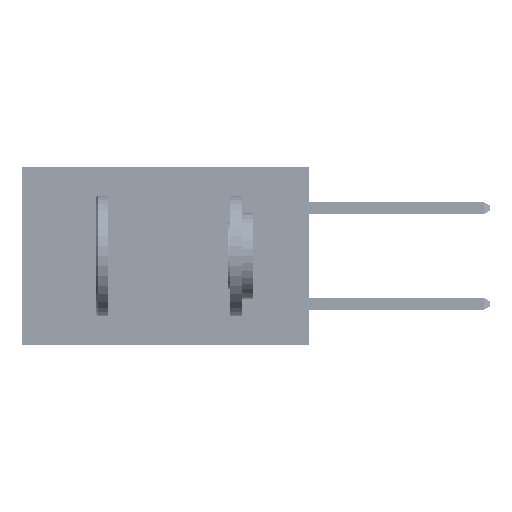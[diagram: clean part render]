
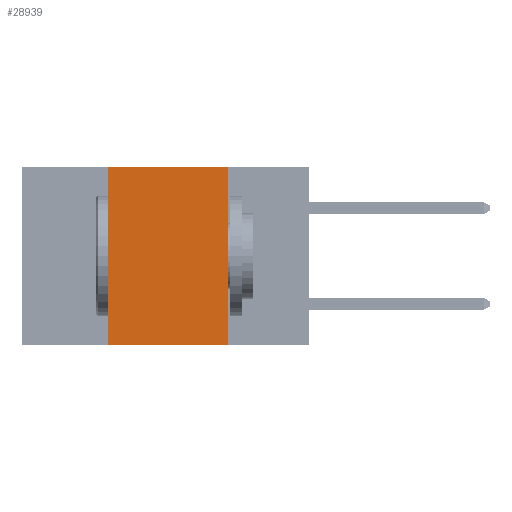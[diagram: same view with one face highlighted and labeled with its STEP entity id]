
A CAD part, left-side view. The second image highlights one B-rep face of the part: STEP entity #28939.
In plain terms, the highlighted planar face has unit normal (-1, 0, 0).
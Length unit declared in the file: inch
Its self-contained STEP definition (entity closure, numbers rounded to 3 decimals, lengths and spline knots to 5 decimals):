
#405 = VECTOR ( 'NONE', #922, 39.37008 ) ;
#922 = DIRECTION ( 'NONE',  ( 0., 0., 1. ) ) ;
#2161 = EDGE_LOOP ( 'NONE', ( #22562, #3399, #42289, #28009 ) ) ;
#2400 = DIRECTION ( 'NONE',  ( 0., -1., 0. ) ) ;
#3399 = ORIENTED_EDGE ( 'NONE', *, *, #45378, .F. ) ;
#3670 = VECTOR ( 'NONE', #2400, 39.37008 ) ;
#4872 = VECTOR ( 'NONE', #13951, 39.37008 ) ;
#6285 = CARTESIAN_POINT ( 'NONE',  ( 0., 0.6, 0. ) ) ;
#7671 = LINE ( 'NONE', #22929, #45826 ) ;
#9110 = AXIS2_PLACEMENT_3D ( 'NONE', #14588, #41474, #18618 ) ;
#10226 = CARTESIAN_POINT ( 'NONE',  ( 0., 0.42, -0.37 ) ) ;
#12044 = CARTESIAN_POINT ( 'NONE',  ( 0., 0.17, -0.37 ) ) ;
#13951 = DIRECTION ( 'NONE',  ( 0., -1., 0. ) ) ;
#14588 = CARTESIAN_POINT ( 'NONE',  ( 0., 0.6, 0. ) ) ;
#14754 = PLANE ( 'NONE',  #9110 ) ;
#15049 = LINE ( 'NONE', #17637, #3670 ) ;
#15059 = LINE ( 'NONE', #6285, #4872 ) ;
#17637 = CARTESIAN_POINT ( 'NONE',  ( 0., 0.6, -0.37 ) ) ;
#18618 = DIRECTION ( 'NONE',  ( 0., 0., -1. ) ) ;
#19259 = DIRECTION ( 'NONE',  ( 0., 0., -1. ) ) ;
#20032 = CARTESIAN_POINT ( 'NONE',  ( 0., 0.42, 0. ) ) ;
#22004 = LINE ( 'NONE', #20032, #405 ) ;
#22562 = ORIENTED_EDGE ( 'NONE', *, *, #41859, .F. ) ;
#22929 = CARTESIAN_POINT ( 'NONE',  ( 0., 0.17, 0. ) ) ;
#23958 = EDGE_CURVE ( 'NONE', #41584, #40954, #22004, .T. ) ;
#27490 = EDGE_CURVE ( 'NONE', #41584, #46346, #15049, .T. ) ;
#28009 = ORIENTED_EDGE ( 'NONE', *, *, #27490, .T. ) ;
#28939 = ADVANCED_FACE ( 'NONE', ( #45161 ), #14754, .F. ) ;
#31730 = CARTESIAN_POINT ( 'NONE',  ( 0., 0.17, 0. ) ) ;
#37484 = CARTESIAN_POINT ( 'NONE',  ( 0., 0.42, 0. ) ) ;
#40954 = VERTEX_POINT ( 'NONE', #37484 ) ;
#41474 = DIRECTION ( 'NONE',  ( 1., 0., 0. ) ) ;
#41584 = VERTEX_POINT ( 'NONE', #10226 ) ;
#41859 = EDGE_CURVE ( 'NONE', #48633, #46346, #7671, .T. ) ;
#42289 = ORIENTED_EDGE ( 'NONE', *, *, #23958, .F. ) ;
#45161 = FACE_OUTER_BOUND ( 'NONE', #2161, .T. ) ;
#45378 = EDGE_CURVE ( 'NONE', #40954, #48633, #15059, .T. ) ;
#45826 = VECTOR ( 'NONE', #19259, 39.37008 ) ;
#46346 = VERTEX_POINT ( 'NONE', #12044 ) ;
#48633 = VERTEX_POINT ( 'NONE', #31730 ) ;
